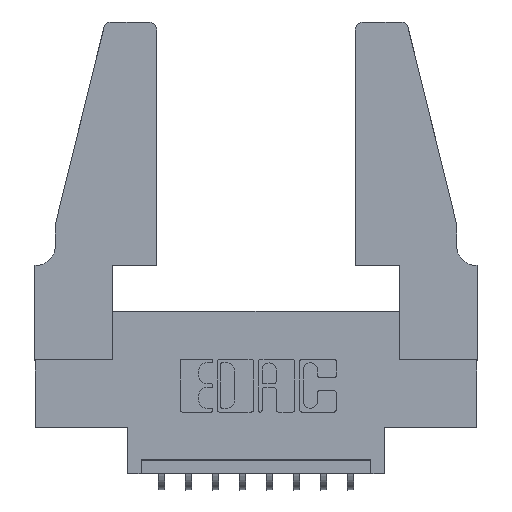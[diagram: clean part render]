
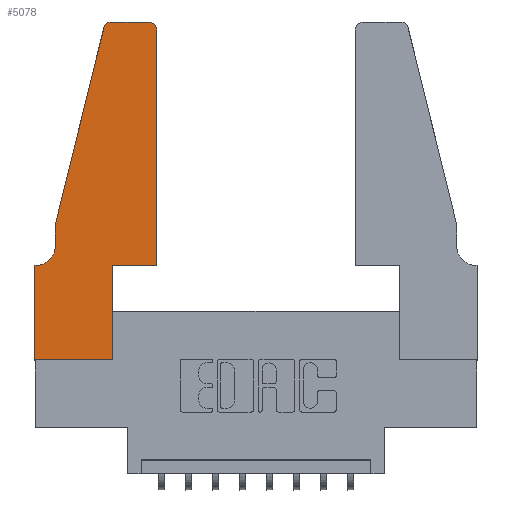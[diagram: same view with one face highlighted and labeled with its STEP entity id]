
A CAD part, top view. The second image highlights one B-rep face of the part: STEP entity #5078.
In plain terms, the highlighted planar face has unit normal (0, 0, 1).
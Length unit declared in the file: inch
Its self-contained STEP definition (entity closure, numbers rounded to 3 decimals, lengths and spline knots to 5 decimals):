
#48 = VERTEX_POINT ( 'NONE', #3503 ) ;
#182 = DIRECTION ( 'NONE',  ( 0., -1., 0. ) ) ;
#337 = LINE ( 'NONE', #1334, #12591 ) ;
#403 = AXIS2_PLACEMENT_3D ( 'NONE', #5236, #3230, #10295 ) ;
#445 = CARTESIAN_POINT ( 'NONE',  ( 0.0055, 0.35, 0.37 ) ) ;
#514 = VECTOR ( 'NONE', #1666, 39.37008 ) ;
#548 = CARTESIAN_POINT ( 'NONE',  ( 0.4505, 1.22, 0.37 ) ) ;
#787 = LINE ( 'NONE', #5594, #12094 ) ;
#847 = DIRECTION ( 'NONE',  ( 0., -1., 0. ) ) ;
#1024 = CARTESIAN_POINT ( 'NONE',  ( 0.0755, 0.5, 0.37 ) ) ;
#1050 = DIRECTION ( 'NONE',  ( 1., 0., 0. ) ) ;
#1186 = CARTESIAN_POINT ( 'NONE',  ( 0.25487, 1.22718, 0.37 ) ) ;
#1330 = CARTESIAN_POINT ( 'NONE',  ( 0.2865, 0.35, 0.37 ) ) ;
#1334 = CARTESIAN_POINT ( 'NONE',  ( 0.0755, 0.5, 0.37 ) ) ;
#1350 = EDGE_CURVE ( 'NONE', #9135, #10046, #787, .T. ) ;
#1359 = VECTOR ( 'NONE', #847, 39.37008 ) ;
#1473 = EDGE_CURVE ( 'NONE', #6230, #9122, #2957, .T. ) ;
#1666 = DIRECTION ( 'NONE',  ( 0., 1., 0. ) ) ;
#1704 = VECTOR ( 'NONE', #182, 39.37008 ) ;
#1722 = DIRECTION ( 'NONE',  ( 0., 0., 1. ) ) ;
#1778 = ORIENTED_EDGE ( 'NONE', *, *, #3144, .T. ) ;
#1817 = EDGE_LOOP ( 'NONE', ( #8310, #7585, #5368, #1778, #11632, #7582, #3422, #2692, #8622, #10949, #6629, #6651 ) ) ;
#2305 = CARTESIAN_POINT ( 'NONE',  ( 0.284, 1.22, 0.37 ) ) ;
#2351 = LINE ( 'NONE', #3007, #10111 ) ;
#2373 = CARTESIAN_POINT ( 'NONE',  ( 0.4505, 0.35, 0.37 ) ) ;
#2417 = DIRECTION ( 'NONE',  ( 1., 0., 0. ) ) ;
#2511 = EDGE_CURVE ( 'NONE', #48, #2740, #7467, .T. ) ;
#2528 = VECTOR ( 'NONE', #2417, 39.37008 ) ;
#2692 = ORIENTED_EDGE ( 'NONE', *, *, #10418, .T. ) ;
#2740 = VERTEX_POINT ( 'NONE', #7235 ) ;
#2773 = CARTESIAN_POINT ( 'NONE',  ( 0.4205, 1.25, 0.37 ) ) ;
#2957 = LINE ( 'NONE', #12734, #12866 ) ;
#3007 = CARTESIAN_POINT ( 'NONE',  ( 0., 0., 0.37 ) ) ;
#3144 = EDGE_CURVE ( 'NONE', #4747, #4925, #4530, .T. ) ;
#3230 = DIRECTION ( 'NONE',  ( 0., 0., 1. ) ) ;
#3317 = DIRECTION ( 'NONE',  ( 1., 0., 0. ) ) ;
#3422 = ORIENTED_EDGE ( 'NONE', *, *, #2511, .T. ) ;
#3503 = CARTESIAN_POINT ( 'NONE',  ( 0., 0.35, 0.37 ) ) ;
#3520 = CARTESIAN_POINT ( 'NONE',  ( 0.2865, 0., 0.37 ) ) ;
#3566 = DIRECTION ( 'NONE',  ( -1., 0., 0. ) ) ;
#3952 = CIRCLE ( 'NONE', #7937, 0.03 ) ;
#4331 = EDGE_CURVE ( 'NONE', #9122, #5841, #9409, .T. ) ;
#4530 = LINE ( 'NONE', #1024, #1704 ) ;
#4631 = VERTEX_POINT ( 'NONE', #548 ) ;
#4747 = VERTEX_POINT ( 'NONE', #12966 ) ;
#4925 = VERTEX_POINT ( 'NONE', #8173 ) ;
#5078 = ADVANCED_FACE ( 'NONE', ( #5621 ), #7183, .T. ) ;
#5236 = CARTESIAN_POINT ( 'NONE',  ( 0., 0.35, 0.37 ) ) ;
#5368 = ORIENTED_EDGE ( 'NONE', *, *, #10431, .T. ) ;
#5594 = CARTESIAN_POINT ( 'NONE',  ( 0.2865, 0.35, 0.37 ) ) ;
#5621 = FACE_OUTER_BOUND ( 'NONE', #1817, .T. ) ;
#5841 = VERTEX_POINT ( 'NONE', #1186 ) ;
#6230 = VERTEX_POINT ( 'NONE', #2773 ) ;
#6417 = DIRECTION ( 'NONE',  ( 0., 1., 0. ) ) ;
#6606 = LINE ( 'NONE', #7400, #514 ) ;
#6629 = ORIENTED_EDGE ( 'NONE', *, *, #10245, .T. ) ;
#6651 = ORIENTED_EDGE ( 'NONE', *, *, #11406, .T. ) ;
#7045 = VERTEX_POINT ( 'NONE', #445 ) ;
#7183 = PLANE ( 'NONE',  #403 ) ;
#7235 = CARTESIAN_POINT ( 'NONE',  ( 0., 0., 0.37 ) ) ;
#7380 = CARTESIAN_POINT ( 'NONE',  ( 0.0755, 0.35, 0.37 ) ) ;
#7400 = CARTESIAN_POINT ( 'NONE',  ( 0.4505, 0.35, 0.37 ) ) ;
#7437 = AXIS2_PLACEMENT_3D ( 'NONE', #2305, #9351, #3317 ) ;
#7467 = LINE ( 'NONE', #10034, #1359 ) ;
#7512 = DIRECTION ( 'NONE',  ( -1., 0., 0. ) ) ;
#7582 = ORIENTED_EDGE ( 'NONE', *, *, #9145, .T. ) ;
#7585 = ORIENTED_EDGE ( 'NONE', *, *, #4331, .T. ) ;
#7937 = AXIS2_PLACEMENT_3D ( 'NONE', #11715, #1722, #9088 ) ;
#8173 = CARTESIAN_POINT ( 'NONE',  ( 0.0755, 0.42, 0.37 ) ) ;
#8310 = ORIENTED_EDGE ( 'NONE', *, *, #1473, .T. ) ;
#8591 = CARTESIAN_POINT ( 'NONE',  ( 0.284, 1.25, 0.37 ) ) ;
#8622 = ORIENTED_EDGE ( 'NONE', *, *, #1350, .T. ) ;
#9077 = EDGE_CURVE ( 'NONE', #10046, #12908, #12282, .T. ) ;
#9088 = DIRECTION ( 'NONE',  ( 1., 0., 0. ) ) ;
#9122 = VERTEX_POINT ( 'NONE', #8591 ) ;
#9135 = VERTEX_POINT ( 'NONE', #3520 ) ;
#9145 = EDGE_CURVE ( 'NONE', #7045, #48, #9786, .T. ) ;
#9351 = DIRECTION ( 'NONE',  ( 0., 0., 1. ) ) ;
#9409 = CIRCLE ( 'NONE', #7437, 0.03 ) ;
#9417 = DIRECTION ( 'NONE',  ( -0.239, -0.971, 0. ) ) ;
#9786 = LINE ( 'NONE', #7380, #12925 ) ;
#9828 = DIRECTION ( 'NONE',  ( -1., 0., 0. ) ) ;
#9897 = CARTESIAN_POINT ( 'NONE',  ( 0.4505, 0.35, 0.37 ) ) ;
#9922 = EDGE_CURVE ( 'NONE', #4925, #7045, #12143, .T. ) ;
#10034 = CARTESIAN_POINT ( 'NONE',  ( 0., 0., 0.37 ) ) ;
#10046 = VERTEX_POINT ( 'NONE', #1330 ) ;
#10111 = VECTOR ( 'NONE', #1050, 39.37008 ) ;
#10245 = EDGE_CURVE ( 'NONE', #12908, #4631, #6606, .T. ) ;
#10295 = DIRECTION ( 'NONE',  ( 1., 0., 0. ) ) ;
#10418 = EDGE_CURVE ( 'NONE', #2740, #9135, #2351, .T. ) ;
#10431 = EDGE_CURVE ( 'NONE', #5841, #4747, #337, .T. ) ;
#10949 = ORIENTED_EDGE ( 'NONE', *, *, #9077, .T. ) ;
#11358 = CARTESIAN_POINT ( 'NONE',  ( 0.0055, 0.42, 0.37 ) ) ;
#11406 = EDGE_CURVE ( 'NONE', #4631, #6230, #3952, .T. ) ;
#11466 = AXIS2_PLACEMENT_3D ( 'NONE', #11358, #11483, #7512 ) ;
#11483 = DIRECTION ( 'NONE',  ( 0., 0., -1. ) ) ;
#11632 = ORIENTED_EDGE ( 'NONE', *, *, #9922, .T. ) ;
#11715 = CARTESIAN_POINT ( 'NONE',  ( 0.4205, 1.22, 0.37 ) ) ;
#12094 = VECTOR ( 'NONE', #6417, 39.37008 ) ;
#12143 = CIRCLE ( 'NONE', #11466, 0.07 ) ;
#12282 = LINE ( 'NONE', #2373, #2528 ) ;
#12591 = VECTOR ( 'NONE', #9417, 39.37008 ) ;
#12734 = CARTESIAN_POINT ( 'NONE',  ( 0.2605, 1.25, 0.37 ) ) ;
#12866 = VECTOR ( 'NONE', #9828, 39.37008 ) ;
#12908 = VERTEX_POINT ( 'NONE', #9897 ) ;
#12925 = VECTOR ( 'NONE', #3566, 39.37008 ) ;
#12966 = CARTESIAN_POINT ( 'NONE',  ( 0.0755, 0.5, 0.37 ) ) ;
